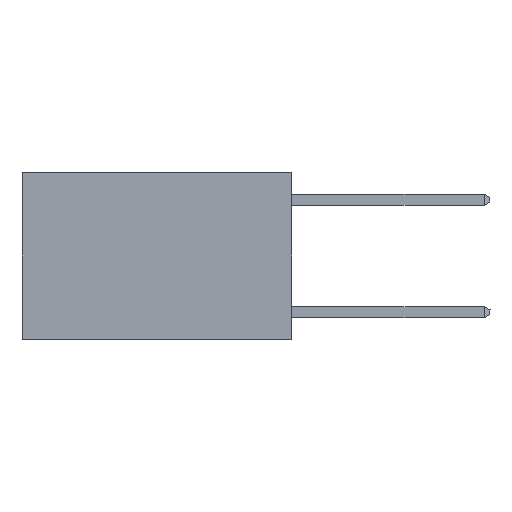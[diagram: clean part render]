
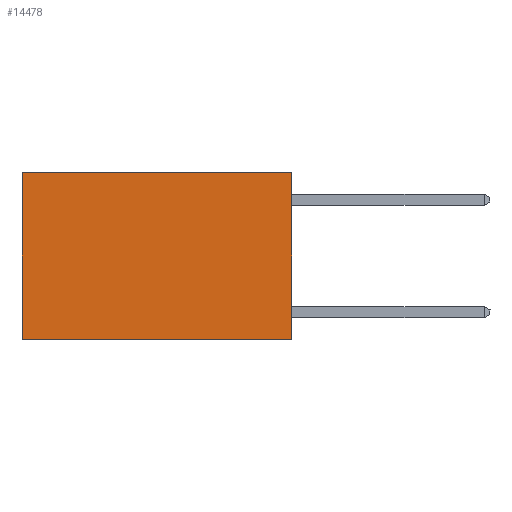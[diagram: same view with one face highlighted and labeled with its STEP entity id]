
A CAD part, left-side view. The second image highlights one B-rep face of the part: STEP entity #14478.
In plain terms, the highlighted planar face has unit normal (-1, 0, 0).
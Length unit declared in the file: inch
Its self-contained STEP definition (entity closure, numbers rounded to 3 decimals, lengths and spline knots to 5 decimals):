
#126 = AXIS2_PLACEMENT_3D ( 'NONE', #21514, #11408, #592 ) ;
#592 = DIRECTION ( 'NONE',  ( 0., 0., -1. ) ) ;
#877 = CARTESIAN_POINT ( 'NONE',  ( 0.2625, 0., -0.37 ) ) ;
#1059 = CARTESIAN_POINT ( 'NONE',  ( 0.2625, 0.6, 0. ) ) ;
#1835 = ORIENTED_EDGE ( 'NONE', *, *, #7322, .T. ) ;
#4359 = ORIENTED_EDGE ( 'NONE', *, *, #16517, .T. ) ;
#7322 = EDGE_CURVE ( 'NONE', #20058, #9468, #18647, .T. ) ;
#7895 = PLANE ( 'NONE',  #126 ) ;
#8159 = VECTOR ( 'NONE', #9097, 39.37008 ) ;
#8255 = CARTESIAN_POINT ( 'NONE',  ( 0.2625, 0.6, -0.37 ) ) ;
#9097 = DIRECTION ( 'NONE',  ( 0., 1., 0. ) ) ;
#9468 = VERTEX_POINT ( 'NONE', #15726 ) ;
#10016 = VECTOR ( 'NONE', #11897, 39.37008 ) ;
#11408 = DIRECTION ( 'NONE',  ( 1., 0., 0. ) ) ;
#11412 = LINE ( 'NONE', #1059, #11947 ) ;
#11556 = ORIENTED_EDGE ( 'NONE', *, *, #11695, .F. ) ;
#11695 = EDGE_CURVE ( 'NONE', #20058, #13956, #22352, .T. ) ;
#11823 = ORIENTED_EDGE ( 'NONE', *, *, #20956, .F. ) ;
#11897 = DIRECTION ( 'NONE',  ( 0., 0., -1. ) ) ;
#11947 = VECTOR ( 'NONE', #20308, 39.37008 ) ;
#12773 = LINE ( 'NONE', #19363, #8159 ) ;
#13856 = DIRECTION ( 'NONE',  ( 0., 1., 0. ) ) ;
#13956 = VERTEX_POINT ( 'NONE', #877 ) ;
#14137 = VECTOR ( 'NONE', #13856, 39.37008 ) ;
#14478 = ADVANCED_FACE ( 'NONE', ( #21771 ), #7895, .F. ) ;
#15726 = CARTESIAN_POINT ( 'NONE',  ( 0.2625, 0.6, 0. ) ) ;
#16517 = EDGE_CURVE ( 'NONE', #9468, #21288, #11412, .T. ) ;
#16940 = CARTESIAN_POINT ( 'NONE',  ( 0.2625, 0., 0. ) ) ;
#17507 = EDGE_LOOP ( 'NONE', ( #4359, #11823, #11556, #1835 ) ) ;
#18647 = LINE ( 'NONE', #20610, #14137 ) ;
#19363 = CARTESIAN_POINT ( 'NONE',  ( 0.2625, 0., -0.37 ) ) ;
#20058 = VERTEX_POINT ( 'NONE', #16940 ) ;
#20308 = DIRECTION ( 'NONE',  ( 0., 0., -1. ) ) ;
#20359 = CARTESIAN_POINT ( 'NONE',  ( 0.2625, 0., 0. ) ) ;
#20610 = CARTESIAN_POINT ( 'NONE',  ( 0.2625, 0., 0. ) ) ;
#20956 = EDGE_CURVE ( 'NONE', #13956, #21288, #12773, .T. ) ;
#21288 = VERTEX_POINT ( 'NONE', #8255 ) ;
#21514 = CARTESIAN_POINT ( 'NONE',  ( 0.2625, 0., 0. ) ) ;
#21771 = FACE_OUTER_BOUND ( 'NONE', #17507, .T. ) ;
#22352 = LINE ( 'NONE', #20359, #10016 ) ;
